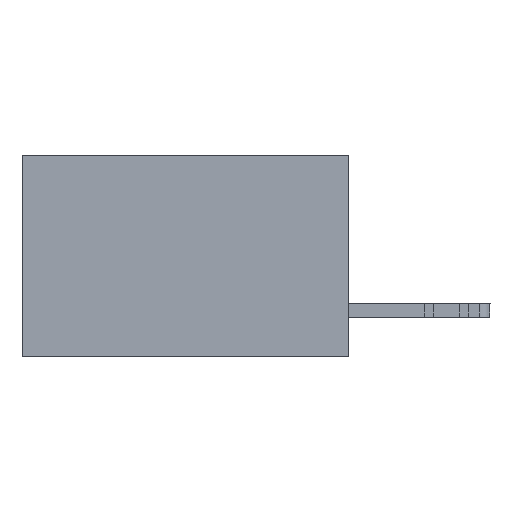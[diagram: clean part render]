
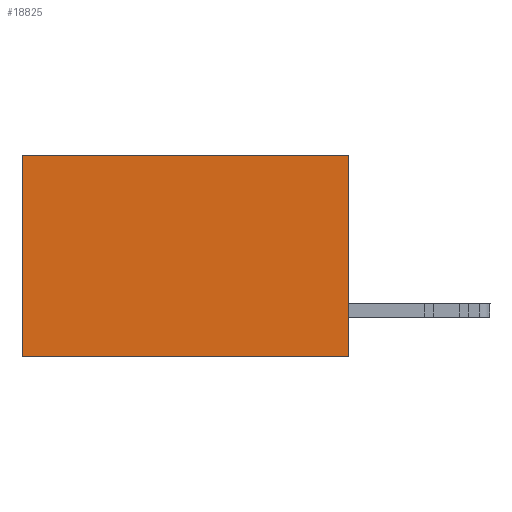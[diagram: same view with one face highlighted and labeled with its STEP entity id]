
A CAD part, left-side view. The second image highlights one B-rep face of the part: STEP entity #18825.
In plain terms, the highlighted planar face has unit normal (-1, 0, 0).
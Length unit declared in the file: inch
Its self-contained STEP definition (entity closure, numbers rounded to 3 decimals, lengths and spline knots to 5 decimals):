
#705 = DIRECTION ( 'NONE',  ( 0., 1., 0. ) ) ;
#1234 = CARTESIAN_POINT ( 'NONE',  ( 0.2615, 0., -0.37 ) ) ;
#1537 = VERTEX_POINT ( 'NONE', #21499 ) ;
#2620 = CARTESIAN_POINT ( 'NONE',  ( 0.2615, 0.6, -0.37 ) ) ;
#3620 = ORIENTED_EDGE ( 'NONE', *, *, #6470, .T. ) ;
#3778 = CARTESIAN_POINT ( 'NONE',  ( 0.2615, 0., -0.37 ) ) ;
#4370 = DIRECTION ( 'NONE',  ( 0., 0., -1. ) ) ;
#4534 = ORIENTED_EDGE ( 'NONE', *, *, #24647, .F. ) ;
#4668 = DIRECTION ( 'NONE',  ( 0., 1., 0. ) ) ;
#5086 = EDGE_CURVE ( 'NONE', #1537, #6824, #20342, .T. ) ;
#5814 = VECTOR ( 'NONE', #4668, 39.37008 ) ;
#6328 = CARTESIAN_POINT ( 'NONE',  ( 0.2615, 0.6, -0.37 ) ) ;
#6452 = VECTOR ( 'NONE', #4370, 39.37008 ) ;
#6470 = EDGE_CURVE ( 'NONE', #6824, #15023, #8699, .T. ) ;
#6824 = VERTEX_POINT ( 'NONE', #25399 ) ;
#8269 = EDGE_CURVE ( 'NONE', #1537, #12330, #23396, .T. ) ;
#8699 = LINE ( 'NONE', #6328, #6452 ) ;
#9114 = PLANE ( 'NONE',  #12875 ) ;
#10816 = CARTESIAN_POINT ( 'NONE',  ( 0.2615, 0., -0.37 ) ) ;
#12330 = VERTEX_POINT ( 'NONE', #10816 ) ;
#12875 = AXIS2_PLACEMENT_3D ( 'NONE', #17054, #24102, #19668 ) ;
#14678 = ORIENTED_EDGE ( 'NONE', *, *, #8269, .F. ) ;
#14801 = ORIENTED_EDGE ( 'NONE', *, *, #5086, .T. ) ;
#14935 = LINE ( 'NONE', #1234, #16930 ) ;
#15023 = VERTEX_POINT ( 'NONE', #2620 ) ;
#16500 = VECTOR ( 'NONE', #23770, 39.37008 ) ;
#16930 = VECTOR ( 'NONE', #705, 39.37008 ) ;
#17054 = CARTESIAN_POINT ( 'NONE',  ( 0.2615, 0., -0.37 ) ) ;
#18825 = ADVANCED_FACE ( 'NONE', ( #19001 ), #9114, .F. ) ;
#19001 = FACE_OUTER_BOUND ( 'NONE', #21671, .T. ) ;
#19668 = DIRECTION ( 'NONE',  ( 0., 0., -1. ) ) ;
#20342 = LINE ( 'NONE', #22589, #5814 ) ;
#21499 = CARTESIAN_POINT ( 'NONE',  ( 0.2615, 0., 0. ) ) ;
#21671 = EDGE_LOOP ( 'NONE', ( #3620, #4534, #14678, #14801 ) ) ;
#22589 = CARTESIAN_POINT ( 'NONE',  ( 0.2615, 0., 0. ) ) ;
#23396 = LINE ( 'NONE', #3778, #16500 ) ;
#23770 = DIRECTION ( 'NONE',  ( 0., 0., -1. ) ) ;
#24102 = DIRECTION ( 'NONE',  ( 1., 0., 0. ) ) ;
#24647 = EDGE_CURVE ( 'NONE', #12330, #15023, #14935, .T. ) ;
#25399 = CARTESIAN_POINT ( 'NONE',  ( 0.2615, 0.6, 0. ) ) ;
